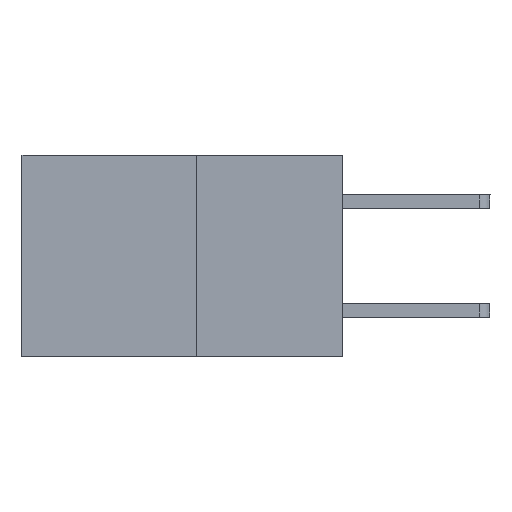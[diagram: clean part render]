
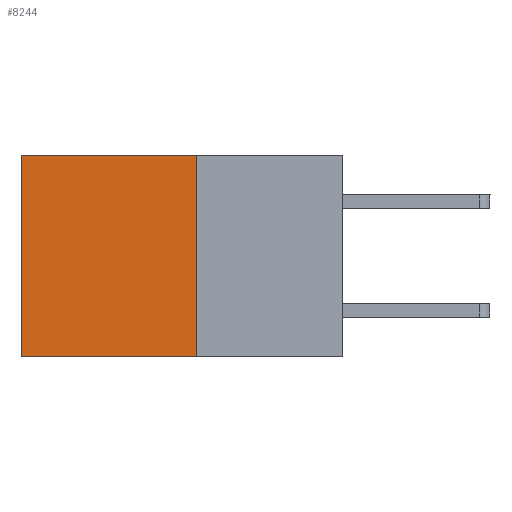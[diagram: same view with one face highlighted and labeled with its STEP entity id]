
A CAD part, left-side view. The second image highlights one B-rep face of the part: STEP entity #8244.
In plain terms, the highlighted planar face has unit normal (-1, 0, 0).
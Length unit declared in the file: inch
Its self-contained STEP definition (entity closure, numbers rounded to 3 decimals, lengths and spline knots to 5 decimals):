
#178 = CARTESIAN_POINT ( 'NONE',  ( 0.277, 0.27, 0. ) ) ;
#394 = CARTESIAN_POINT ( 'NONE',  ( 0.277, 0.27, -0.37 ) ) ;
#854 = ORIENTED_EDGE ( 'NONE', *, *, #8716, .T. ) ;
#2642 = EDGE_CURVE ( 'NONE', #6810, #10150, #4196, .T. ) ;
#2884 = VECTOR ( 'NONE', #6890, 39.37008 ) ;
#3085 = LINE ( 'NONE', #8801, #2884 ) ;
#3411 = DIRECTION ( 'NONE',  ( 1., 0., 0. ) ) ;
#4196 = LINE ( 'NONE', #394, #8957 ) ;
#5029 = LINE ( 'NONE', #8869, #12382 ) ;
#5150 = CARTESIAN_POINT ( 'NONE',  ( 0.277, 0.27, -0.37 ) ) ;
#5279 = PLANE ( 'NONE',  #9112 ) ;
#5343 = FACE_OUTER_BOUND ( 'NONE', #8178, .T. ) ;
#6072 = CARTESIAN_POINT ( 'NONE',  ( 0.277, 0.27, -0.37 ) ) ;
#6079 = EDGE_CURVE ( 'NONE', #12071, #6810, #11965, .T. ) ;
#6754 = CARTESIAN_POINT ( 'NONE',  ( 0.277, 0.59, -0.37 ) ) ;
#6795 = DIRECTION ( 'NONE',  ( 0., 0., -1. ) ) ;
#6810 = VERTEX_POINT ( 'NONE', #9536 ) ;
#6890 = DIRECTION ( 'NONE',  ( 0., 1., 0. ) ) ;
#6964 = DIRECTION ( 'NONE',  ( 0., 0., -1. ) ) ;
#7338 = VERTEX_POINT ( 'NONE', #10778 ) ;
#8178 = EDGE_LOOP ( 'NONE', ( #9403, #9758, #10801, #854 ) ) ;
#8188 = EDGE_CURVE ( 'NONE', #7338, #10150, #5029, .T. ) ;
#8211 = DIRECTION ( 'NONE',  ( 0., 1., 0. ) ) ;
#8244 = ADVANCED_FACE ( 'NONE', ( #5343 ), #5279, .F. ) ;
#8716 = EDGE_CURVE ( 'NONE', #12071, #7338, #3085, .T. ) ;
#8801 = CARTESIAN_POINT ( 'NONE',  ( 0.277, 0.27, 0. ) ) ;
#8869 = CARTESIAN_POINT ( 'NONE',  ( 0.277, 0.59, -0.37 ) ) ;
#8957 = VECTOR ( 'NONE', #8211, 39.37008 ) ;
#9112 = AXIS2_PLACEMENT_3D ( 'NONE', #5150, #3411, #6964 ) ;
#9403 = ORIENTED_EDGE ( 'NONE', *, *, #8188, .T. ) ;
#9536 = CARTESIAN_POINT ( 'NONE',  ( 0.277, 0.27, -0.37 ) ) ;
#9758 = ORIENTED_EDGE ( 'NONE', *, *, #2642, .F. ) ;
#10150 = VERTEX_POINT ( 'NONE', #6754 ) ;
#10778 = CARTESIAN_POINT ( 'NONE',  ( 0.277, 0.59, 0. ) ) ;
#10801 = ORIENTED_EDGE ( 'NONE', *, *, #6079, .F. ) ;
#11108 = VECTOR ( 'NONE', #11836, 39.37008 ) ;
#11836 = DIRECTION ( 'NONE',  ( 0., 0., -1. ) ) ;
#11965 = LINE ( 'NONE', #6072, #11108 ) ;
#12071 = VERTEX_POINT ( 'NONE', #178 ) ;
#12382 = VECTOR ( 'NONE', #6795, 39.37008 ) ;
